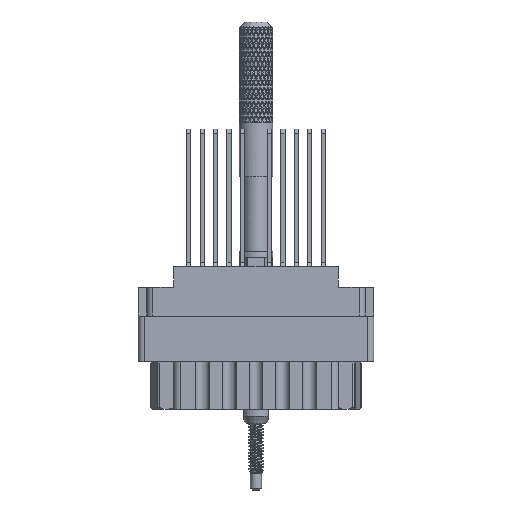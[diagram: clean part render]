
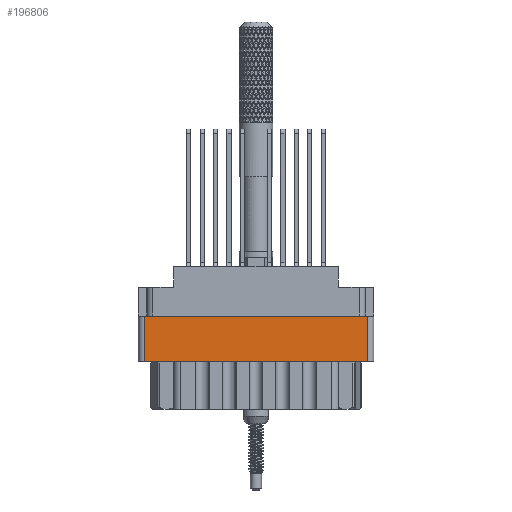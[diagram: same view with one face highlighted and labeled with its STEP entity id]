
A CAD part, front view. The second image highlights one B-rep face of the part: STEP entity #196806.
In plain terms, the highlighted planar face has unit normal (0, -1, 0).
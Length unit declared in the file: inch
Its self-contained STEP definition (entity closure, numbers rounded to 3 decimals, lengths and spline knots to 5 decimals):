
#7909 = CARTESIAN_POINT ( 'NONE',  ( 0., -0.343, -0.277 ) ) ;
#17423 = VERTEX_POINT ( 'NONE', #167692 ) ;
#18164 = ORIENTED_EDGE ( 'NONE', *, *, #186797, .F. ) ;
#25251 = DIRECTION ( 'NONE',  ( 0., 0., 1. ) ) ;
#29584 = EDGE_LOOP ( 'NONE', ( #79481, #126559, #18164, #29985 ) ) ;
#29985 = ORIENTED_EDGE ( 'NONE', *, *, #92937, .T. ) ;
#37543 = VERTEX_POINT ( 'NONE', #109158 ) ;
#37777 = VERTEX_POINT ( 'NONE', #77175 ) ;
#56284 = CARTESIAN_POINT ( 'NONE',  ( -0.624, -0.343, -0.798 ) ) ;
#57247 = PLANE ( 'NONE',  #101424 ) ;
#70389 = VECTOR ( 'NONE', #172361, 39.37008 ) ;
#75159 = LINE ( 'NONE', #78957, #70389 ) ;
#75757 = LINE ( 'NONE', #117499, #78058 ) ;
#76629 = CARTESIAN_POINT ( 'NONE',  ( 0.624, -0.343, -0.277 ) ) ;
#77175 = CARTESIAN_POINT ( 'NONE',  ( 0.624, -0.343, -0.529 ) ) ;
#78058 = VECTOR ( 'NONE', #25251, 39.37008 ) ;
#78957 = CARTESIAN_POINT ( 'NONE',  ( 0., -0.343, -0.529 ) ) ;
#79192 = VECTOR ( 'NONE', #177546, 39.37008 ) ;
#79481 = ORIENTED_EDGE ( 'NONE', *, *, #149237, .F. ) ;
#92937 = EDGE_CURVE ( 'NONE', #37777, #105169, #75757, .T. ) ;
#100487 = EDGE_CURVE ( 'NONE', #17423, #37543, #181102, .T. ) ;
#101424 = AXIS2_PLACEMENT_3D ( 'NONE', #132209, #132875, #115650 ) ;
#104770 = LINE ( 'NONE', #7909, #140392 ) ;
#105169 = VERTEX_POINT ( 'NONE', #76629 ) ;
#109158 = CARTESIAN_POINT ( 'NONE',  ( -0.624, -0.343, -0.529 ) ) ;
#115650 = DIRECTION ( 'NONE',  ( 0., 0., -1. ) ) ;
#117499 = CARTESIAN_POINT ( 'NONE',  ( 0.624, -0.343, -0.798 ) ) ;
#118838 = FACE_OUTER_BOUND ( 'NONE', #29584, .T. ) ;
#126559 = ORIENTED_EDGE ( 'NONE', *, *, #100487, .T. ) ;
#128139 = DIRECTION ( 'NONE',  ( 1., 0., 0. ) ) ;
#132209 = CARTESIAN_POINT ( 'NONE',  ( -0.656, -0.343, -0.798 ) ) ;
#132875 = DIRECTION ( 'NONE',  ( 0., -1., 0. ) ) ;
#140392 = VECTOR ( 'NONE', #128139, 39.37008 ) ;
#149237 = EDGE_CURVE ( 'NONE', #17423, #105169, #104770, .T. ) ;
#167692 = CARTESIAN_POINT ( 'NONE',  ( -0.624, -0.343, -0.277 ) ) ;
#172361 = DIRECTION ( 'NONE',  ( -1., 0., 0. ) ) ;
#177546 = DIRECTION ( 'NONE',  ( 0., 0., -1. ) ) ;
#181102 = LINE ( 'NONE', #56284, #79192 ) ;
#186797 = EDGE_CURVE ( 'NONE', #37777, #37543, #75159, .T. ) ;
#196806 = ADVANCED_FACE ( 'NONE', ( #118838 ), #57247, .T. ) ;
